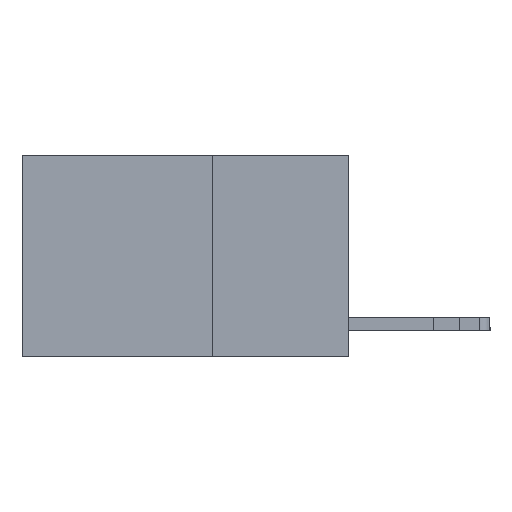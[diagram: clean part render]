
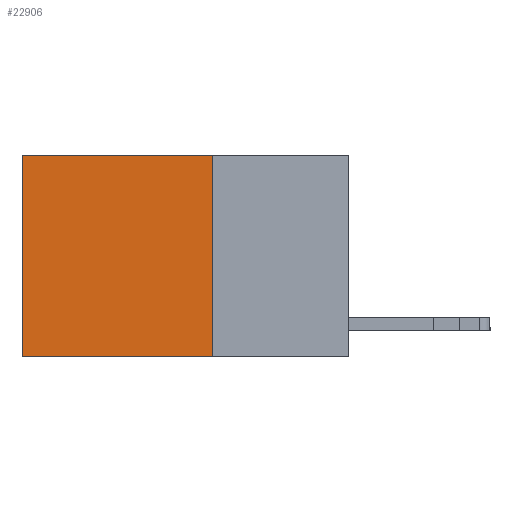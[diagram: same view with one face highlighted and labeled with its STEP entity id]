
A CAD part, left-side view. The second image highlights one B-rep face of the part: STEP entity #22906.
In plain terms, the highlighted planar face has unit normal (-1, 0, 0).
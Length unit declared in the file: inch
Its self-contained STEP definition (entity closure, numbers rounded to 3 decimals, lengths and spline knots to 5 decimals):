
#373 = LINE ( 'NONE', #3586, #4719 ) ;
#795 = CARTESIAN_POINT ( 'NONE',  ( 0.2625, 0.6, 0. ) ) ;
#1902 = CARTESIAN_POINT ( 'NONE',  ( 0.2625, 0.25, 0. ) ) ;
#2952 = DIRECTION ( 'NONE',  ( 0., 0., -1. ) ) ;
#3234 = EDGE_CURVE ( 'NONE', #18059, #6783, #9658, .T. ) ;
#3586 = CARTESIAN_POINT ( 'NONE',  ( 0.2625, 0.25, -0.37 ) ) ;
#4559 = ORIENTED_EDGE ( 'NONE', *, *, #3234, .T. ) ;
#4719 = VECTOR ( 'NONE', #21846, 39.37008 ) ;
#5906 = VECTOR ( 'NONE', #12859, 39.37008 ) ;
#6050 = CARTESIAN_POINT ( 'NONE',  ( 0.2625, 0.25, 0. ) ) ;
#6783 = VERTEX_POINT ( 'NONE', #12876 ) ;
#7460 = LINE ( 'NONE', #1902, #5906 ) ;
#9001 = PLANE ( 'NONE',  #10030 ) ;
#9658 = LINE ( 'NONE', #15397, #16840 ) ;
#10030 = AXIS2_PLACEMENT_3D ( 'NONE', #19383, #17976, #23032 ) ;
#11330 = EDGE_LOOP ( 'NONE', ( #16503, #12983, #18097, #4559 ) ) ;
#11768 = VERTEX_POINT ( 'NONE', #22160 ) ;
#12668 = VERTEX_POINT ( 'NONE', #20183 ) ;
#12859 = DIRECTION ( 'NONE',  ( 0., 0., -1. ) ) ;
#12876 = CARTESIAN_POINT ( 'NONE',  ( 0.2625, 0.6, 0. ) ) ;
#12983 = ORIENTED_EDGE ( 'NONE', *, *, #14023, .F. ) ;
#14023 = EDGE_CURVE ( 'NONE', #11768, #12668, #373, .T. ) ;
#15397 = CARTESIAN_POINT ( 'NONE',  ( 0.2625, 0.25, 0. ) ) ;
#16503 = ORIENTED_EDGE ( 'NONE', *, *, #20546, .T. ) ;
#16840 = VECTOR ( 'NONE', #22480, 39.37008 ) ;
#17976 = DIRECTION ( 'NONE',  ( 1., 0., 0. ) ) ;
#18059 = VERTEX_POINT ( 'NONE', #6050 ) ;
#18097 = ORIENTED_EDGE ( 'NONE', *, *, #23092, .F. ) ;
#19383 = CARTESIAN_POINT ( 'NONE',  ( 0.2625, 0.25, 0. ) ) ;
#19824 = VECTOR ( 'NONE', #2952, 39.37008 ) ;
#20183 = CARTESIAN_POINT ( 'NONE',  ( 0.2625, 0.6, -0.37 ) ) ;
#20546 = EDGE_CURVE ( 'NONE', #6783, #12668, #22396, .T. ) ;
#21499 = FACE_OUTER_BOUND ( 'NONE', #11330, .T. ) ;
#21846 = DIRECTION ( 'NONE',  ( 0., 1., 0. ) ) ;
#22160 = CARTESIAN_POINT ( 'NONE',  ( 0.2625, 0.25, -0.37 ) ) ;
#22396 = LINE ( 'NONE', #795, #19824 ) ;
#22480 = DIRECTION ( 'NONE',  ( 0., 1., 0. ) ) ;
#22906 = ADVANCED_FACE ( 'NONE', ( #21499 ), #9001, .F. ) ;
#23032 = DIRECTION ( 'NONE',  ( 0., 0., -1. ) ) ;
#23092 = EDGE_CURVE ( 'NONE', #18059, #11768, #7460, .T. ) ;
